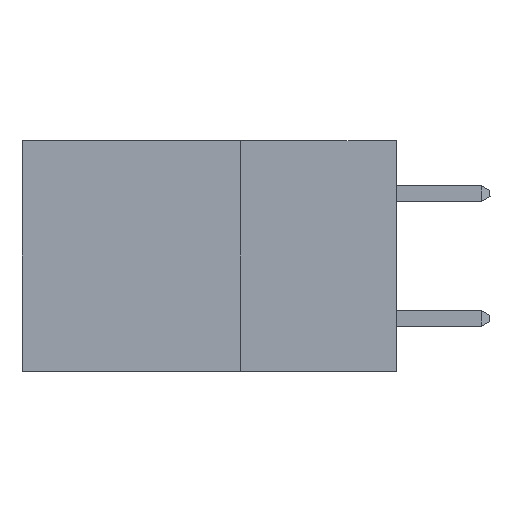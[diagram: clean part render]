
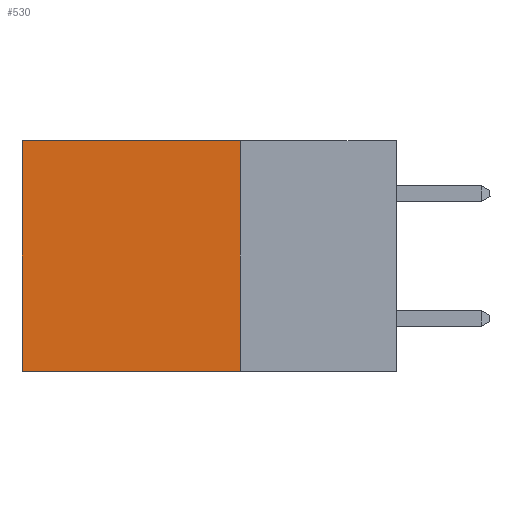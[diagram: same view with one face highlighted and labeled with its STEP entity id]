
A CAD part, left-side view. The second image highlights one B-rep face of the part: STEP entity #530.
In plain terms, the highlighted planar face has unit normal (-1, 0, 0).
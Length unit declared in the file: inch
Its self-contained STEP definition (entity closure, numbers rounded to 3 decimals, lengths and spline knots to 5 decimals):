
#188 = VERTEX_POINT ( 'NONE', #12794 ) ;
#530 = ADVANCED_FACE ( 'NONE', ( #11342 ), #6977, .F. ) ;
#1318 = VERTEX_POINT ( 'NONE', #13286 ) ;
#1403 = DIRECTION ( 'NONE',  ( 0., 0., -1. ) ) ;
#1872 = EDGE_CURVE ( 'NONE', #2666, #188, #17933, .T. ) ;
#2666 = VERTEX_POINT ( 'NONE', #13527 ) ;
#2888 = EDGE_CURVE ( 'NONE', #3836, #2666, #14943, .T. ) ;
#2909 = LINE ( 'NONE', #15817, #7085 ) ;
#3836 = VERTEX_POINT ( 'NONE', #13948 ) ;
#3855 = LINE ( 'NONE', #7823, #14677 ) ;
#4637 = EDGE_CURVE ( 'NONE', #1318, #188, #3855, .T. ) ;
#5668 = ORIENTED_EDGE ( 'NONE', *, *, #8712, .T. ) ;
#6540 = EDGE_LOOP ( 'NONE', ( #8372, #15721, #10368, #5668 ) ) ;
#6948 = DIRECTION ( 'NONE',  ( 0., 1., 0. ) ) ;
#6977 = PLANE ( 'NONE',  #17837 ) ;
#7085 = VECTOR ( 'NONE', #11531, 39.37008 ) ;
#7823 = CARTESIAN_POINT ( 'NONE',  ( 0.298, 0.6, 0. ) ) ;
#8317 = VECTOR ( 'NONE', #1403, 39.37008 ) ;
#8372 = ORIENTED_EDGE ( 'NONE', *, *, #4637, .T. ) ;
#8712 = EDGE_CURVE ( 'NONE', #3836, #1318, #2909, .T. ) ;
#10159 = DIRECTION ( 'NONE',  ( 1., 0., 0. ) ) ;
#10368 = ORIENTED_EDGE ( 'NONE', *, *, #2888, .F. ) ;
#10394 = VECTOR ( 'NONE', #6948, 39.37008 ) ;
#11261 = CARTESIAN_POINT ( 'NONE',  ( 0.298, 0.25, -0.37 ) ) ;
#11342 = FACE_OUTER_BOUND ( 'NONE', #6540, .T. ) ;
#11531 = DIRECTION ( 'NONE',  ( 0., 1., 0. ) ) ;
#12794 = CARTESIAN_POINT ( 'NONE',  ( 0.298, 0.6, -0.37 ) ) ;
#13286 = CARTESIAN_POINT ( 'NONE',  ( 0.298, 0.6, 0. ) ) ;
#13527 = CARTESIAN_POINT ( 'NONE',  ( 0.298, 0.25, -0.37 ) ) ;
#13948 = CARTESIAN_POINT ( 'NONE',  ( 0.298, 0.25, 0. ) ) ;
#14149 = CARTESIAN_POINT ( 'NONE',  ( 0.298, 0.25, 0. ) ) ;
#14390 = CARTESIAN_POINT ( 'NONE',  ( 0.298, 0.25, 0. ) ) ;
#14677 = VECTOR ( 'NONE', #17590, 39.37008 ) ;
#14943 = LINE ( 'NONE', #14149, #8317 ) ;
#15625 = DIRECTION ( 'NONE',  ( 0., 0., -1. ) ) ;
#15721 = ORIENTED_EDGE ( 'NONE', *, *, #1872, .F. ) ;
#15817 = CARTESIAN_POINT ( 'NONE',  ( 0.298, 0.25, 0. ) ) ;
#17590 = DIRECTION ( 'NONE',  ( 0., 0., -1. ) ) ;
#17837 = AXIS2_PLACEMENT_3D ( 'NONE', #14390, #10159, #15625 ) ;
#17933 = LINE ( 'NONE', #11261, #10394 ) ;
